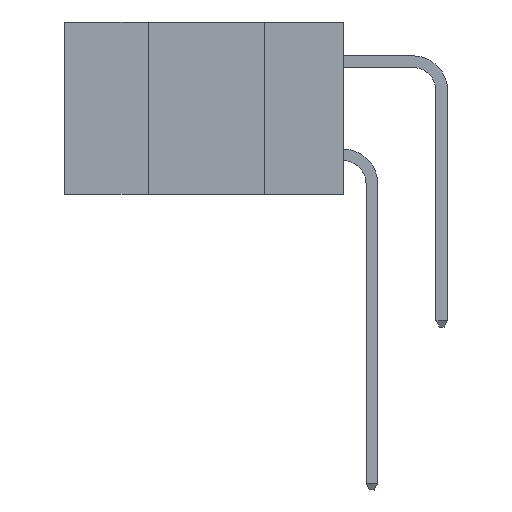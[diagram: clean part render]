
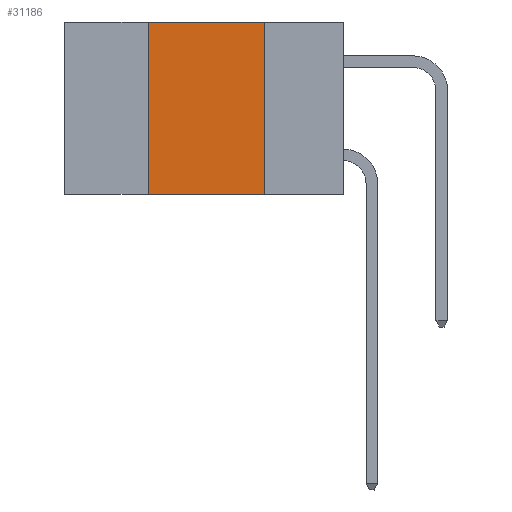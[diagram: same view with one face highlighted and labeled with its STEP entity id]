
A CAD part, left-side view. The second image highlights one B-rep face of the part: STEP entity #31186.
In plain terms, the highlighted planar face has unit normal (-1, 0, 0).
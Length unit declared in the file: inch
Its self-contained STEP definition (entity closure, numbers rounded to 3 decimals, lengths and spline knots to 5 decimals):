
#1849 = VECTOR ( 'NONE', #28115, 39.37008 ) ;
#2101 = CARTESIAN_POINT ( 'NONE',  ( 0., 0.17, -0.37 ) ) ;
#2835 = VECTOR ( 'NONE', #12343, 39.37008 ) ;
#3782 = ORIENTED_EDGE ( 'NONE', *, *, #27398, .F. ) ;
#3812 = EDGE_CURVE ( 'NONE', #19555, #16697, #8546, .T. ) ;
#5000 = CARTESIAN_POINT ( 'NONE',  ( 0., 0.6, 0. ) ) ;
#6504 = EDGE_CURVE ( 'NONE', #19555, #7516, #16687, .T. ) ;
#7516 = VERTEX_POINT ( 'NONE', #17653 ) ;
#8546 = LINE ( 'NONE', #24427, #21366 ) ;
#8664 = FACE_OUTER_BOUND ( 'NONE', #15241, .T. ) ;
#9864 = DIRECTION ( 'NONE',  ( 0., 0., -1. ) ) ;
#9930 = CARTESIAN_POINT ( 'NONE',  ( 0., 0.6, 0. ) ) ;
#10268 = VECTOR ( 'NONE', #21238, 39.37008 ) ;
#12343 = DIRECTION ( 'NONE',  ( 0., -1., 0. ) ) ;
#14864 = ORIENTED_EDGE ( 'NONE', *, *, #30482, .F. ) ;
#15241 = EDGE_LOOP ( 'NONE', ( #3782, #14864, #19590, #25483 ) ) ;
#16687 = LINE ( 'NONE', #28408, #10268 ) ;
#16697 = VERTEX_POINT ( 'NONE', #2101 ) ;
#17653 = CARTESIAN_POINT ( 'NONE',  ( 0., 0.42, 0. ) ) ;
#19555 = VERTEX_POINT ( 'NONE', #21480 ) ;
#19590 = ORIENTED_EDGE ( 'NONE', *, *, #6504, .F. ) ;
#21180 = LINE ( 'NONE', #23275, #1849 ) ;
#21238 = DIRECTION ( 'NONE',  ( 0., 0., 1. ) ) ;
#21366 = VECTOR ( 'NONE', #26688, 39.37008 ) ;
#21480 = CARTESIAN_POINT ( 'NONE',  ( 0., 0.42, -0.37 ) ) ;
#21910 = PLANE ( 'NONE',  #29289 ) ;
#22166 = LINE ( 'NONE', #9930, #2835 ) ;
#23275 = CARTESIAN_POINT ( 'NONE',  ( 0., 0.17, 0. ) ) ;
#24357 = DIRECTION ( 'NONE',  ( 1., 0., 0. ) ) ;
#24427 = CARTESIAN_POINT ( 'NONE',  ( 0., 0.6, -0.37 ) ) ;
#25483 = ORIENTED_EDGE ( 'NONE', *, *, #3812, .T. ) ;
#26688 = DIRECTION ( 'NONE',  ( 0., -1., 0. ) ) ;
#27398 = EDGE_CURVE ( 'NONE', #29680, #16697, #21180, .T. ) ;
#28115 = DIRECTION ( 'NONE',  ( 0., 0., -1. ) ) ;
#28408 = CARTESIAN_POINT ( 'NONE',  ( 0., 0.42, 0. ) ) ;
#28744 = CARTESIAN_POINT ( 'NONE',  ( 0., 0.17, 0. ) ) ;
#29289 = AXIS2_PLACEMENT_3D ( 'NONE', #5000, #24357, #9864 ) ;
#29680 = VERTEX_POINT ( 'NONE', #28744 ) ;
#30482 = EDGE_CURVE ( 'NONE', #7516, #29680, #22166, .T. ) ;
#31186 = ADVANCED_FACE ( 'NONE', ( #8664 ), #21910, .F. ) ;
